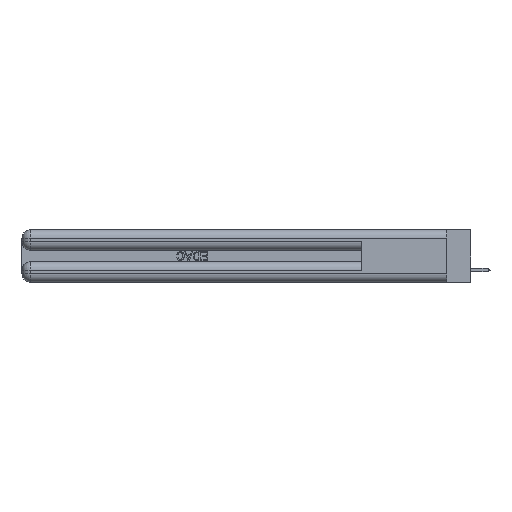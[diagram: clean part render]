
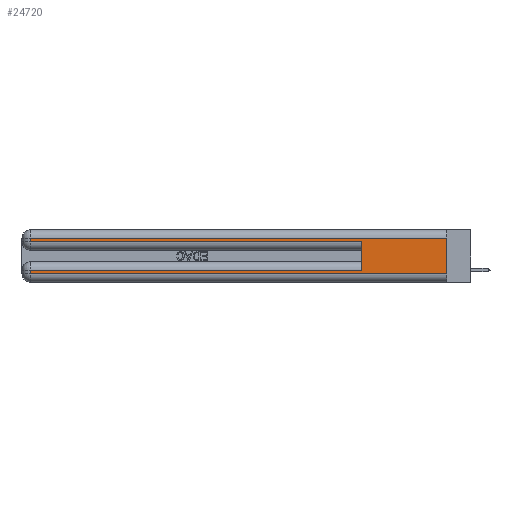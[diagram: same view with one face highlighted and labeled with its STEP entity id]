
A CAD part, left-side view. The second image highlights one B-rep face of the part: STEP entity #24720.
In plain terms, the highlighted planar face has unit normal (-1, 0, 0).
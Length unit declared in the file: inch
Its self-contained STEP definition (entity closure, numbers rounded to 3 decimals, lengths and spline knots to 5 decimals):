
#1287 = EDGE_CURVE ( 'NONE', #43551, #1814, #20325, .T. ) ;
#1814 = VERTEX_POINT ( 'NONE', #50382 ) ;
#2118 = DIRECTION ( 'NONE',  ( 0., 1., 0. ) ) ;
#2533 = AXIS2_PLACEMENT_3D ( 'NONE', #34722, #10847, #43420 ) ;
#2987 = VERTEX_POINT ( 'NONE', #14461 ) ;
#4227 = ORIENTED_EDGE ( 'NONE', *, *, #45560, .F. ) ;
#4866 = EDGE_CURVE ( 'NONE', #6905, #2987, #45385, .T. ) ;
#5195 = DIRECTION ( 'NONE',  ( 0., 0., -1. ) ) ;
#6534 = DIRECTION ( 'NONE',  ( 0., 0., -1. ) ) ;
#6681 = CARTESIAN_POINT ( 'NONE',  ( 0., 0., 0.285 ) ) ;
#6905 = VERTEX_POINT ( 'NONE', #39099 ) ;
#7823 = EDGE_LOOP ( 'NONE', ( #4227, #27071, #33803, #45027, #8010, #41377, #23959, #13466 ) ) ;
#8010 = ORIENTED_EDGE ( 'NONE', *, *, #36047, .F. ) ;
#8964 = VECTOR ( 'NONE', #31109, 39.37008 ) ;
#9112 = LINE ( 'NONE', #44868, #37016 ) ;
#10847 = DIRECTION ( 'NONE',  ( 1., 0., 0. ) ) ;
#11226 = DIRECTION ( 'NONE',  ( 0., -1., 0. ) ) ;
#12618 = FACE_OUTER_BOUND ( 'NONE', #7823, .T. ) ;
#13466 = ORIENTED_EDGE ( 'NONE', *, *, #20680, .T. ) ;
#13670 = CARTESIAN_POINT ( 'NONE',  ( 0., 0., 0.06 ) ) ;
#14461 = CARTESIAN_POINT ( 'NONE',  ( 0., 2.94, 0.06 ) ) ;
#15268 = VERTEX_POINT ( 'NONE', #38694 ) ;
#15899 = EDGE_CURVE ( 'NONE', #35574, #43551, #19181, .T. ) ;
#19181 = LINE ( 'NONE', #36354, #31863 ) ;
#19469 = VECTOR ( 'NONE', #6534, 39.37008 ) ;
#20325 = LINE ( 'NONE', #6681, #8964 ) ;
#20562 = DIRECTION ( 'NONE',  ( 0., 1., 0. ) ) ;
#20680 = EDGE_CURVE ( 'NONE', #2987, #44264, #44252, .T. ) ;
#22261 = CARTESIAN_POINT ( 'NONE',  ( 0., 0., 0.085 ) ) ;
#22392 = CARTESIAN_POINT ( 'NONE',  ( 0., 2.94, 0.37 ) ) ;
#23114 = LINE ( 'NONE', #22261, #49657 ) ;
#23204 = PLANE ( 'NONE',  #2533 ) ;
#23959 = ORIENTED_EDGE ( 'NONE', *, *, #4866, .T. ) ;
#24720 = ADVANCED_FACE ( 'NONE', ( #12618 ), #23204, .F. ) ;
#25309 = CARTESIAN_POINT ( 'NONE',  ( 0., 0., 0.06 ) ) ;
#25752 = VECTOR ( 'NONE', #11226, 39.37008 ) ;
#27071 = ORIENTED_EDGE ( 'NONE', *, *, #44102, .T. ) ;
#27452 = CARTESIAN_POINT ( 'NONE',  ( 0., 0.6, 0.145 ) ) ;
#30043 = CARTESIAN_POINT ( 'NONE',  ( 0., 0., 0.37 ) ) ;
#30136 = CARTESIAN_POINT ( 'NONE',  ( 0., 2.94, 0.31 ) ) ;
#31109 = DIRECTION ( 'NONE',  ( 0., -1., 0. ) ) ;
#31791 = VECTOR ( 'NONE', #34170, 39.37008 ) ;
#31863 = VECTOR ( 'NONE', #5195, 39.37008 ) ;
#33650 = LINE ( 'NONE', #30043, #31791 ) ;
#33803 = ORIENTED_EDGE ( 'NONE', *, *, #15899, .T. ) ;
#34170 = DIRECTION ( 'NONE',  ( 0., 0., -1. ) ) ;
#34722 = CARTESIAN_POINT ( 'NONE',  ( 0., 0., 0.37 ) ) ;
#35574 = VERTEX_POINT ( 'NONE', #30136 ) ;
#36047 = EDGE_CURVE ( 'NONE', #15268, #1814, #42072, .T. ) ;
#36354 = CARTESIAN_POINT ( 'NONE',  ( 0., 2.94, 0.37 ) ) ;
#37016 = VECTOR ( 'NONE', #20562, 39.37008 ) ;
#38694 = CARTESIAN_POINT ( 'NONE',  ( 0., 0.6, 0.085 ) ) ;
#39099 = CARTESIAN_POINT ( 'NONE',  ( 0., 2.94, 0.085 ) ) ;
#40605 = CARTESIAN_POINT ( 'NONE',  ( 0., 0., 0.31 ) ) ;
#41377 = ORIENTED_EDGE ( 'NONE', *, *, #47568, .T. ) ;
#42072 = LINE ( 'NONE', #27452, #49023 ) ;
#43420 = DIRECTION ( 'NONE',  ( 0., 0., -1. ) ) ;
#43551 = VERTEX_POINT ( 'NONE', #49790 ) ;
#44102 = EDGE_CURVE ( 'NONE', #48738, #35574, #9112, .T. ) ;
#44252 = LINE ( 'NONE', #25309, #25752 ) ;
#44264 = VERTEX_POINT ( 'NONE', #13670 ) ;
#44868 = CARTESIAN_POINT ( 'NONE',  ( 0., 0., 0.31 ) ) ;
#45027 = ORIENTED_EDGE ( 'NONE', *, *, #1287, .T. ) ;
#45385 = LINE ( 'NONE', #22392, #19469 ) ;
#45560 = EDGE_CURVE ( 'NONE', #48738, #44264, #33650, .T. ) ;
#47568 = EDGE_CURVE ( 'NONE', #15268, #6905, #23114, .T. ) ;
#47644 = DIRECTION ( 'NONE',  ( 0., 0., 1. ) ) ;
#48738 = VERTEX_POINT ( 'NONE', #40605 ) ;
#49023 = VECTOR ( 'NONE', #47644, 39.37008 ) ;
#49657 = VECTOR ( 'NONE', #2118, 39.37008 ) ;
#49790 = CARTESIAN_POINT ( 'NONE',  ( 0., 2.94, 0.285 ) ) ;
#50382 = CARTESIAN_POINT ( 'NONE',  ( 0., 0.6, 0.285 ) ) ;
